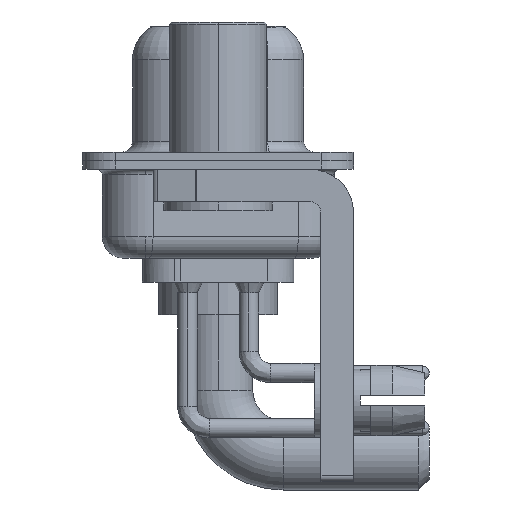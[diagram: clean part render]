
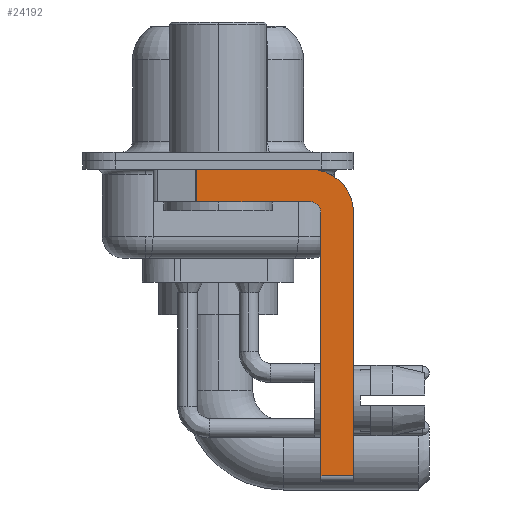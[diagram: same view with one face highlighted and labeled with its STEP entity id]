
A CAD part, left-side view. The second image highlights one B-rep face of the part: STEP entity #24192.
In plain terms, the highlighted planar face has unit normal (-1, 0, 0).
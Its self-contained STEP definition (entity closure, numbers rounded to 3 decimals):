
#562 = ORIENTED_EDGE ( 'NONE', *, *, #11247, .T. ) ;
#715 = VERTEX_POINT ( 'NONE', #8204 ) ;
#1084 = VERTEX_POINT ( 'NONE', #17867 ) ;
#1092 = CARTESIAN_POINT ( 'NONE',  ( -2.9, -4.75, -14.8 ) ) ;
#2991 = CARTESIAN_POINT ( 'NONE',  ( -2.9, -4.25, -1.9 ) ) ;
#3087 = CARTESIAN_POINT ( 'NONE',  ( -2.9, 0.978, -1.9 ) ) ;
#3410 = CARTESIAN_POINT ( 'NONE',  ( -2.9, -4.25, -14.55 ) ) ;
#5460 = ORIENTED_EDGE ( 'NONE', *, *, #17616, .F. ) ;
#5782 = DIRECTION ( 'NONE',  ( 1., 0., 0. ) ) ;
#6225 = ORIENTED_EDGE ( 'NONE', *, *, #24965, .T. ) ;
#6405 = ORIENTED_EDGE ( 'NONE', *, *, #13948, .F. ) ;
#6547 = ORIENTED_EDGE ( 'NONE', *, *, #16422, .F. ) ;
#6643 = CARTESIAN_POINT ( 'NONE',  ( -2.9, -6.25, -14.55 ) ) ;
#7000 = LINE ( 'NONE', #20926, #11056 ) ;
#7229 = EDGE_CURVE ( 'NONE', #18000, #25507, #15509, .T. ) ;
#7332 = CIRCLE ( 'NONE', #13696, 2. ) ;
#7788 = EDGE_CURVE ( 'NONE', #25507, #715, #7332, .T. ) ;
#7814 = DIRECTION ( 'NONE',  ( 0., -1., 0. ) ) ;
#8186 = DIRECTION ( 'NONE',  ( 0., 0., -1. ) ) ;
#8204 = CARTESIAN_POINT ( 'NONE',  ( -2.9, -6.25, -2.4 ) ) ;
#8528 = EDGE_CURVE ( 'NONE', #22181, #1084, #18765, .T. ) ;
#8701 = CARTESIAN_POINT ( 'NONE',  ( -2.9, 0.978, -0.4 ) ) ;
#9258 = CARTESIAN_POINT ( 'NONE',  ( -2.9, -4.25, -0.4 ) ) ;
#9392 = LINE ( 'NONE', #2991, #17187 ) ;
#9981 = VERTEX_POINT ( 'NONE', #3087 ) ;
#10123 = ORIENTED_EDGE ( 'NONE', *, *, #8528, .F. ) ;
#10712 = DIRECTION ( 'NONE',  ( 0., 0., 1. ) ) ;
#11056 = VECTOR ( 'NONE', #12973, 1000. ) ;
#11247 = EDGE_CURVE ( 'NONE', #18000, #9981, #7000, .T. ) ;
#12115 = CARTESIAN_POINT ( 'NONE',  ( -2.9, -4.25, -2.4 ) ) ;
#12405 = VECTOR ( 'NONE', #7814, 1000. ) ;
#12435 = DIRECTION ( 'NONE',  ( -1., 0., 0. ) ) ;
#12973 = DIRECTION ( 'NONE',  ( 0., 0., -1. ) ) ;
#13259 = LINE ( 'NONE', #3410, #24982 ) ;
#13291 = VECTOR ( 'NONE', #8186, 1000. ) ;
#13696 = AXIS2_PLACEMENT_3D ( 'NONE', #14027, #5782, #25940 ) ;
#13948 = EDGE_CURVE ( 'NONE', #715, #24453, #18407, .T. ) ;
#14027 = CARTESIAN_POINT ( 'NONE',  ( -2.9, -4.25, -2.4 ) ) ;
#14111 = DIRECTION ( 'NONE',  ( 1., 0., 0. ) ) ;
#14119 = CARTESIAN_POINT ( 'NONE',  ( -2.9, -4.25, -1.9 ) ) ;
#14197 = AXIS2_PLACEMENT_3D ( 'NONE', #16800, #12435, #10712 ) ;
#14229 = PLANE ( 'NONE',  #15219 ) ;
#14352 = FACE_OUTER_BOUND ( 'NONE', #24935, .T. ) ;
#15219 = AXIS2_PLACEMENT_3D ( 'NONE', #12115, #14111, #21918 ) ;
#15509 = LINE ( 'NONE', #15779, #12405 ) ;
#15626 = ORIENTED_EDGE ( 'NONE', *, *, #7788, .F. ) ;
#15779 = CARTESIAN_POINT ( 'NONE',  ( -2.9, 3., -0.4 ) ) ;
#16018 = CARTESIAN_POINT ( 'NONE',  ( -2.9, -6.25, -2.4 ) ) ;
#16422 = EDGE_CURVE ( 'NONE', #1084, #18328, #25605, .T. ) ;
#16631 = DIRECTION ( 'NONE',  ( 0., 0., 1. ) ) ;
#16800 = CARTESIAN_POINT ( 'NONE',  ( -2.9, -4.25, -2.4 ) ) ;
#17187 = VECTOR ( 'NONE', #19203, 1000. ) ;
#17616 = EDGE_CURVE ( 'NONE', #18328, #9981, #9392, .T. ) ;
#17867 = CARTESIAN_POINT ( 'NONE',  ( -2.9, -4.75, -2.4 ) ) ;
#18000 = VERTEX_POINT ( 'NONE', #8701 ) ;
#18328 = VERTEX_POINT ( 'NONE', #14119 ) ;
#18407 = LINE ( 'NONE', #16018, #13291 ) ;
#18765 = LINE ( 'NONE', #1092, #24950 ) ;
#19203 = DIRECTION ( 'NONE',  ( 0., 1., 0. ) ) ;
#20926 = CARTESIAN_POINT ( 'NONE',  ( -2.9, 0.978, -1.9 ) ) ;
#21342 = DIRECTION ( 'NONE',  ( 0., -1., 0. ) ) ;
#21918 = DIRECTION ( 'NONE',  ( 0., 0., -1. ) ) ;
#22181 = VERTEX_POINT ( 'NONE', #24257 ) ;
#24192 = ADVANCED_FACE ( 'NONE', ( #14352 ), #14229, .F. ) ;
#24257 = CARTESIAN_POINT ( 'NONE',  ( -2.9, -4.75, -14.55 ) ) ;
#24453 = VERTEX_POINT ( 'NONE', #6643 ) ;
#24935 = EDGE_LOOP ( 'NONE', ( #25344, #562, #5460, #6547, #10123, #6225, #6405, #15626 ) ) ;
#24950 = VECTOR ( 'NONE', #16631, 1000. ) ;
#24965 = EDGE_CURVE ( 'NONE', #22181, #24453, #13259, .T. ) ;
#24982 = VECTOR ( 'NONE', #21342, 1000. ) ;
#25344 = ORIENTED_EDGE ( 'NONE', *, *, #7229, .F. ) ;
#25507 = VERTEX_POINT ( 'NONE', #9258 ) ;
#25605 = CIRCLE ( 'NONE', #14197, 0.5 ) ;
#25940 = DIRECTION ( 'NONE',  ( 0., 0., -1. ) ) ;
